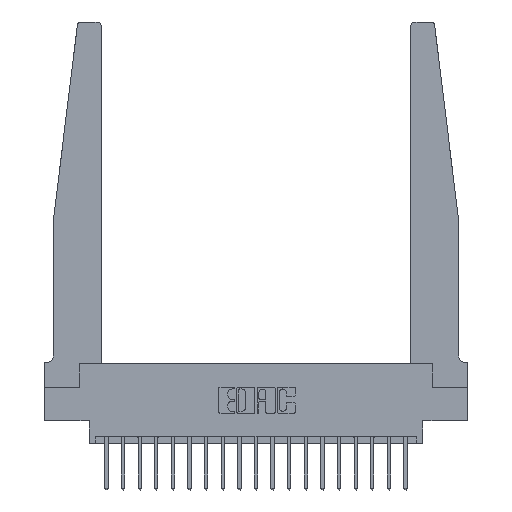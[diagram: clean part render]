
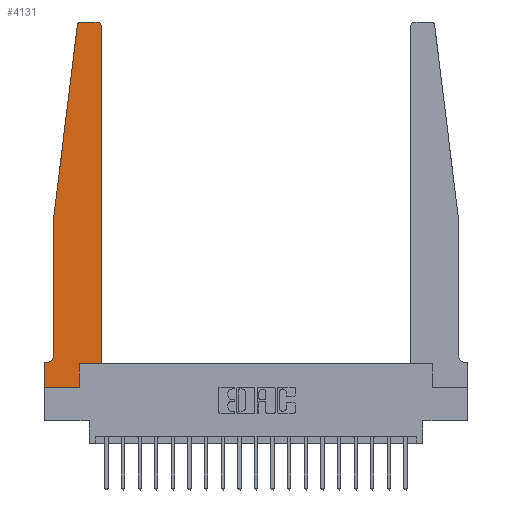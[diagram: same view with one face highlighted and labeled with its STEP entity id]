
A CAD part, top view. The second image highlights one B-rep face of the part: STEP entity #4131.
In plain terms, the highlighted planar face has unit normal (0, 0, 1).
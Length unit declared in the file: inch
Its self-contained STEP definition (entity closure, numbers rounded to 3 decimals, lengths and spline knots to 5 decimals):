
#78 = VERTEX_POINT ( 'NONE', #3747 ) ;
#116 = ORIENTED_EDGE ( 'NONE', *, *, #4461, .T. ) ;
#406 = VERTEX_POINT ( 'NONE', #18831 ) ;
#597 = VECTOR ( 'NONE', #7285, 39.37008 ) ;
#612 = LINE ( 'NONE', #11002, #18413 ) ;
#844 = DIRECTION ( 'NONE',  ( 1., 0., 0. ) ) ;
#1461 = FACE_OUTER_BOUND ( 'NONE', #3535, .T. ) ;
#1554 = CARTESIAN_POINT ( 'NONE',  ( 0.27653, 2.72, 0.37 ) ) ;
#1586 = VERTEX_POINT ( 'NONE', #14007 ) ;
#1620 = AXIS2_PLACEMENT_3D ( 'NONE', #12259, #2833, #13854 ) ;
#1657 = EDGE_CURVE ( 'NONE', #8079, #19412, #6959, .T. ) ;
#1700 = ORIENTED_EDGE ( 'NONE', *, *, #11307, .T. ) ;
#1726 = LINE ( 'NONE', #10179, #9618 ) ;
#1861 = VERTEX_POINT ( 'NONE', #5167 ) ;
#2095 = VECTOR ( 'NONE', #16665, 39.37008 ) ;
#2107 = AXIS2_PLACEMENT_3D ( 'NONE', #1554, #12572, #3138 ) ;
#2322 = DIRECTION ( 'NONE',  ( 0., 1., 0. ) ) ;
#2680 = VERTEX_POINT ( 'NONE', #2954 ) ;
#2833 = DIRECTION ( 'NONE',  ( 0., 0., -1. ) ) ;
#2954 = CARTESIAN_POINT ( 'NONE',  ( 0., 0., 0.37 ) ) ;
#3117 = DIRECTION ( 'NONE',  ( -0.122, -0.992, 0. ) ) ;
#3138 = DIRECTION ( 'NONE',  ( 1., 0., 0. ) ) ;
#3168 = DIRECTION ( 'NONE',  ( 1., 0., 0. ) ) ;
#3535 = EDGE_LOOP ( 'NONE', ( #12261, #18070, #6795, #19057, #116, #5640, #8298, #11864, #17288, #14933, #19342, #1700 ) ) ;
#3747 = CARTESIAN_POINT ( 'NONE',  ( 0.425, 0.18, 0.37 ) ) ;
#4072 = CARTESIAN_POINT ( 'NONE',  ( 0.425, 0.18, 0.37 ) ) ;
#4131 = ADVANCED_FACE ( 'NONE', ( #1461 ), #16198, .T. ) ;
#4461 = EDGE_CURVE ( 'NONE', #10922, #406, #7457, .T. ) ;
#4565 = CARTESIAN_POINT ( 'NONE',  ( 0.425, 2.72, 0.37 ) ) ;
#4793 = LINE ( 'NONE', #13561, #597 ) ;
#5167 = CARTESIAN_POINT ( 'NONE',  ( 0.2605, 0., 0.37 ) ) ;
#5398 = DIRECTION ( 'NONE',  ( -1., 0., 0. ) ) ;
#5491 = EDGE_CURVE ( 'NONE', #78, #10800, #1726, .T. ) ;
#5640 = ORIENTED_EDGE ( 'NONE', *, *, #15963, .T. ) ;
#5791 = AXIS2_PLACEMENT_3D ( 'NONE', #19738, #10281, #844 ) ;
#5891 = EDGE_CURVE ( 'NONE', #19412, #10922, #19986, .T. ) ;
#6005 = CARTESIAN_POINT ( 'NONE',  ( 0.27653, 2.75, 0.37 ) ) ;
#6348 = CARTESIAN_POINT ( 'NONE',  ( 0.065, 0.2375, 0.37 ) ) ;
#6368 = CARTESIAN_POINT ( 'NONE',  ( 0.065, 0.1875, 0.37 ) ) ;
#6509 = CARTESIAN_POINT ( 'NONE',  ( 0.395, 2.75, 0.37 ) ) ;
#6767 = CARTESIAN_POINT ( 'NONE',  ( 0., 0.1875, 0.37 ) ) ;
#6795 = ORIENTED_EDGE ( 'NONE', *, *, #1657, .T. ) ;
#6959 = LINE ( 'NONE', #10964, #14839 ) ;
#7285 = DIRECTION ( 'NONE',  ( 0., -1., 0. ) ) ;
#7298 = AXIS2_PLACEMENT_3D ( 'NONE', #6767, #8335, #19386 ) ;
#7323 = VECTOR ( 'NONE', #7949, 39.37008 ) ;
#7457 = CIRCLE ( 'NONE', #1620, 0.05 ) ;
#7893 = EDGE_CURVE ( 'NONE', #16663, #8811, #15701, .T. ) ;
#7949 = DIRECTION ( 'NONE',  ( -1., 0., 0. ) ) ;
#8021 = DIRECTION ( 'NONE',  ( 0., -1., 0. ) ) ;
#8079 = VERTEX_POINT ( 'NONE', #12159 ) ;
#8298 = ORIENTED_EDGE ( 'NONE', *, *, #17504, .T. ) ;
#8335 = DIRECTION ( 'NONE',  ( 0., 0., 1. ) ) ;
#8811 = VERTEX_POINT ( 'NONE', #6005 ) ;
#8896 = CIRCLE ( 'NONE', #2107, 0.03 ) ;
#9618 = VECTOR ( 'NONE', #2322, 39.37008 ) ;
#10179 = CARTESIAN_POINT ( 'NONE',  ( 0.425, 0.18, 0.37 ) ) ;
#10281 = DIRECTION ( 'NONE',  ( 0., 0., 1. ) ) ;
#10800 = VERTEX_POINT ( 'NONE', #4565 ) ;
#10906 = EDGE_CURVE ( 'NONE', #1861, #1586, #12402, .T. ) ;
#10922 = VERTEX_POINT ( 'NONE', #6348 ) ;
#10964 = CARTESIAN_POINT ( 'NONE',  ( 0.065, 1.25, 0.37 ) ) ;
#11002 = CARTESIAN_POINT ( 'NONE',  ( 0., 0., 0.37 ) ) ;
#11003 = LINE ( 'NONE', #6368, #7323 ) ;
#11007 = CARTESIAN_POINT ( 'NONE',  ( 0.2605, 0.18, 0.37 ) ) ;
#11307 = EDGE_CURVE ( 'NONE', #10800, #16663, #12658, .T. ) ;
#11570 = VECTOR ( 'NONE', #8021, 39.37008 ) ;
#11864 = ORIENTED_EDGE ( 'NONE', *, *, #17132, .T. ) ;
#12159 = CARTESIAN_POINT ( 'NONE',  ( 0.24675, 2.72367, 0.37 ) ) ;
#12259 = CARTESIAN_POINT ( 'NONE',  ( 0.015, 0.2375, 0.37 ) ) ;
#12261 = ORIENTED_EDGE ( 'NONE', *, *, #7893, .T. ) ;
#12402 = LINE ( 'NONE', #11007, #20299 ) ;
#12572 = DIRECTION ( 'NONE',  ( 0., 0., 1. ) ) ;
#12658 = CIRCLE ( 'NONE', #5791, 0.03 ) ;
#12703 = EDGE_CURVE ( 'NONE', #8811, #8079, #8896, .T. ) ;
#12840 = CARTESIAN_POINT ( 'NONE',  ( 0.065, 1.25, 0.37 ) ) ;
#13254 = CARTESIAN_POINT ( 'NONE',  ( 0.25, 2.75, 0.37 ) ) ;
#13561 = CARTESIAN_POINT ( 'NONE',  ( 0., 0., 0.37 ) ) ;
#13854 = DIRECTION ( 'NONE',  ( -1., 0., 0. ) ) ;
#14007 = CARTESIAN_POINT ( 'NONE',  ( 0.2605, 0.18, 0.37 ) ) ;
#14839 = VECTOR ( 'NONE', #3117, 39.37008 ) ;
#14933 = ORIENTED_EDGE ( 'NONE', *, *, #17456, .T. ) ;
#15081 = VERTEX_POINT ( 'NONE', #18489 ) ;
#15701 = LINE ( 'NONE', #13254, #19408 ) ;
#15782 = DIRECTION ( 'NONE',  ( 0., 1., 0. ) ) ;
#15963 = EDGE_CURVE ( 'NONE', #406, #15081, #11003, .T. ) ;
#16198 = PLANE ( 'NONE',  #7298 ) ;
#16663 = VERTEX_POINT ( 'NONE', #6509 ) ;
#16665 = DIRECTION ( 'NONE',  ( 1., 0., 0. ) ) ;
#17132 = EDGE_CURVE ( 'NONE', #2680, #1861, #612, .T. ) ;
#17288 = ORIENTED_EDGE ( 'NONE', *, *, #10906, .T. ) ;
#17456 = EDGE_CURVE ( 'NONE', #1586, #78, #18394, .T. ) ;
#17504 = EDGE_CURVE ( 'NONE', #15081, #2680, #4793, .T. ) ;
#18070 = ORIENTED_EDGE ( 'NONE', *, *, #12703, .T. ) ;
#18394 = LINE ( 'NONE', #4072, #2095 ) ;
#18413 = VECTOR ( 'NONE', #3168, 39.37008 ) ;
#18489 = CARTESIAN_POINT ( 'NONE',  ( 0., 0.1875, 0.37 ) ) ;
#18831 = CARTESIAN_POINT ( 'NONE',  ( 0.015, 0.1875, 0.37 ) ) ;
#19057 = ORIENTED_EDGE ( 'NONE', *, *, #5891, .T. ) ;
#19076 = CARTESIAN_POINT ( 'NONE',  ( 0.065, 1.25, 0.37 ) ) ;
#19342 = ORIENTED_EDGE ( 'NONE', *, *, #5491, .T. ) ;
#19386 = DIRECTION ( 'NONE',  ( 1., 0., 0. ) ) ;
#19408 = VECTOR ( 'NONE', #5398, 39.37008 ) ;
#19412 = VERTEX_POINT ( 'NONE', #12840 ) ;
#19738 = CARTESIAN_POINT ( 'NONE',  ( 0.395, 2.72, 0.37 ) ) ;
#19986 = LINE ( 'NONE', #19076, #11570 ) ;
#20299 = VECTOR ( 'NONE', #15782, 39.37008 ) ;
